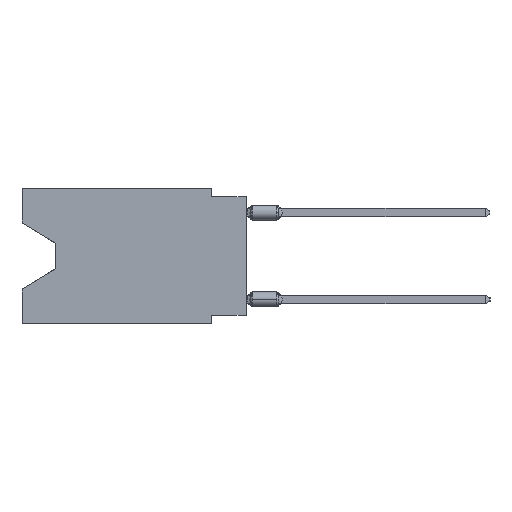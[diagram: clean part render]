
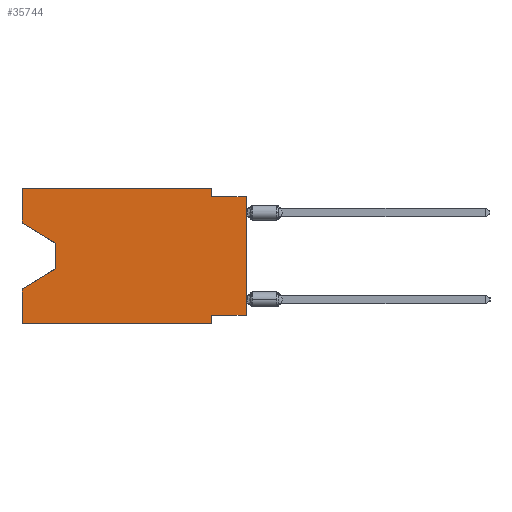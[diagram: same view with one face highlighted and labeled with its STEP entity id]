
A CAD part, left-side view. The second image highlights one B-rep face of the part: STEP entity #35744.
In plain terms, the highlighted planar face has unit normal (-1, 0, 0).
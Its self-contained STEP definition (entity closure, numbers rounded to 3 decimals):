
#128 = DIRECTION ( 'NONE',  ( 0., 1., 0. ) ) ;
#1043 = DIRECTION ( 'NONE',  ( 0., 0., 1. ) ) ;
#1381 = ORIENTED_EDGE ( 'NONE', *, *, #25218, .F. ) ;
#1422 = DIRECTION ( 'NONE',  ( 0., 0., 1. ) ) ;
#1975 = CARTESIAN_POINT ( 'NONE',  ( 0., 2.54, 0. ) ) ;
#2004 = CARTESIAN_POINT ( 'NONE',  ( 0., 16.383, -9.906 ) ) ;
#2198 = VERTEX_POINT ( 'NONE', #19059 ) ;
#2706 = VECTOR ( 'NONE', #7059, 1000. ) ;
#2719 = ORIENTED_EDGE ( 'NONE', *, *, #11180, .F. ) ;
#2769 = VECTOR ( 'NONE', #11578, 1000. ) ;
#6091 = EDGE_CURVE ( 'NONE', #43332, #20529, #32416, .T. ) ;
#7059 = DIRECTION ( 'NONE',  ( 0., -1., 0. ) ) ;
#7175 = VERTEX_POINT ( 'NONE', #13653 ) ;
#8090 = ORIENTED_EDGE ( 'NONE', *, *, #6091, .F. ) ;
#8791 = LINE ( 'NONE', #39538, #25114 ) ;
#9364 = PLANE ( 'NONE',  #44257 ) ;
#9762 = DIRECTION ( 'NONE',  ( 0., -0.855, -0.519 ) ) ;
#10087 = CARTESIAN_POINT ( 'NONE',  ( 0., 0., -0.635 ) ) ;
#10219 = ORIENTED_EDGE ( 'NONE', *, *, #27641, .F. ) ;
#10452 = EDGE_CURVE ( 'NONE', #34812, #7175, #15014, .T. ) ;
#10485 = ORIENTED_EDGE ( 'NONE', *, *, #10452, .F. ) ;
#10496 = VERTEX_POINT ( 'NONE', #26761 ) ;
#10949 = DIRECTION ( 'NONE',  ( 0., 0., -1. ) ) ;
#11180 = EDGE_CURVE ( 'NONE', #10496, #34812, #26831, .T. ) ;
#11578 = DIRECTION ( 'NONE',  ( 0., 0., 1. ) ) ;
#11816 = CARTESIAN_POINT ( 'NONE',  ( 0., 16.383, 0. ) ) ;
#11869 = CARTESIAN_POINT ( 'NONE',  ( 0., 13.97, -5.893 ) ) ;
#12240 = DIRECTION ( 'NONE',  ( 0., 0., -1. ) ) ;
#12267 = EDGE_CURVE ( 'NONE', #14804, #2198, #32508, .T. ) ;
#13176 = EDGE_CURVE ( 'NONE', #7175, #35821, #25823, .T. ) ;
#13653 = CARTESIAN_POINT ( 'NONE',  ( 0., 2.54, -0.635 ) ) ;
#14524 = EDGE_CURVE ( 'NONE', #14804, #10496, #8791, .T. ) ;
#14695 = LINE ( 'NONE', #29933, #27916 ) ;
#14804 = VERTEX_POINT ( 'NONE', #32775 ) ;
#14843 = ORIENTED_EDGE ( 'NONE', *, *, #35526, .T. ) ;
#15014 = LINE ( 'NONE', #19745, #48569 ) ;
#16143 = VECTOR ( 'NONE', #39251, 1000. ) ;
#16859 = CARTESIAN_POINT ( 'NONE',  ( 0., 2.54, -9.271 ) ) ;
#17497 = DIRECTION ( 'NONE',  ( 0., -1., 0. ) ) ;
#17853 = DIRECTION ( 'NONE',  ( 0., 0., -1. ) ) ;
#18412 = CARTESIAN_POINT ( 'NONE',  ( 0., 13.97, -5.893 ) ) ;
#18840 = CARTESIAN_POINT ( 'NONE',  ( 0., 16.383, 0. ) ) ;
#19059 = CARTESIAN_POINT ( 'NONE',  ( 0., 13.97, -4.013 ) ) ;
#19110 = VECTOR ( 'NONE', #128, 1000. ) ;
#19327 = DIRECTION ( 'NONE',  ( 0., -1., 0. ) ) ;
#19745 = CARTESIAN_POINT ( 'NONE',  ( 0., 2.54, 0. ) ) ;
#19930 = CARTESIAN_POINT ( 'NONE',  ( 0., 16.383, 0. ) ) ;
#20529 = VERTEX_POINT ( 'NONE', #24560 ) ;
#20582 = EDGE_LOOP ( 'NONE', ( #40039, #39672, #14843, #8090, #33492, #10219, #1381, #37770, #24499, #10485, #2719, #35408 ) ) ;
#20684 = CARTESIAN_POINT ( 'NONE',  ( 0., 2.54, -9.906 ) ) ;
#20751 = CARTESIAN_POINT ( 'NONE',  ( 0., 2.54, -9.906 ) ) ;
#21979 = VERTEX_POINT ( 'NONE', #23022 ) ;
#22090 = CARTESIAN_POINT ( 'NONE',  ( 0., 0., -0.635 ) ) ;
#22870 = CARTESIAN_POINT ( 'NONE',  ( 0., 0., -9.271 ) ) ;
#23022 = CARTESIAN_POINT ( 'NONE',  ( 0., 0., -9.271 ) ) ;
#24499 = ORIENTED_EDGE ( 'NONE', *, *, #13176, .F. ) ;
#24560 = CARTESIAN_POINT ( 'NONE',  ( 0., 16.383, -7.36 ) ) ;
#25114 = VECTOR ( 'NONE', #1043, 1000. ) ;
#25218 = EDGE_CURVE ( 'NONE', #21979, #26594, #49138, .T. ) ;
#25447 = VECTOR ( 'NONE', #19327, 1000. ) ;
#25823 = LINE ( 'NONE', #10087, #2706 ) ;
#26594 = VERTEX_POINT ( 'NONE', #16859 ) ;
#26761 = CARTESIAN_POINT ( 'NONE',  ( 0., 16.383, 0. ) ) ;
#26831 = LINE ( 'NONE', #11816, #25447 ) ;
#27616 = DIRECTION ( 'NONE',  ( 0., 0.855, -0.519 ) ) ;
#27641 = EDGE_CURVE ( 'NONE', #26594, #38222, #31993, .T. ) ;
#27778 = EDGE_CURVE ( 'NONE', #43332, #38222, #40493, .T. ) ;
#27916 = VECTOR ( 'NONE', #10949, 1000. ) ;
#29819 = CARTESIAN_POINT ( 'NONE',  ( 0., 16.383, -9.906 ) ) ;
#29933 = CARTESIAN_POINT ( 'NONE',  ( 0., 13.97, -4.013 ) ) ;
#30566 = LINE ( 'NONE', #45817, #2769 ) ;
#31354 = LINE ( 'NONE', #11869, #36268 ) ;
#31993 = LINE ( 'NONE', #20751, #16143 ) ;
#32101 = FACE_OUTER_BOUND ( 'NONE', #20582, .T. ) ;
#32416 = LINE ( 'NONE', #19930, #42876 ) ;
#32508 = LINE ( 'NONE', #48500, #44802 ) ;
#32519 = EDGE_CURVE ( 'NONE', #21979, #35821, #30566, .T. ) ;
#32775 = CARTESIAN_POINT ( 'NONE',  ( 0., 16.383, -2.546 ) ) ;
#33492 = ORIENTED_EDGE ( 'NONE', *, *, #27778, .T. ) ;
#34812 = VERTEX_POINT ( 'NONE', #1975 ) ;
#35408 = ORIENTED_EDGE ( 'NONE', *, *, #14524, .F. ) ;
#35526 = EDGE_CURVE ( 'NONE', #38280, #20529, #31354, .T. ) ;
#35744 = ADVANCED_FACE ( 'NONE', ( #32101 ), #9364, .F. ) ;
#35821 = VERTEX_POINT ( 'NONE', #22090 ) ;
#36268 = VECTOR ( 'NONE', #27616, 1000. ) ;
#36894 = VECTOR ( 'NONE', #17497, 1000. ) ;
#37770 = ORIENTED_EDGE ( 'NONE', *, *, #32519, .T. ) ;
#38222 = VERTEX_POINT ( 'NONE', #20684 ) ;
#38280 = VERTEX_POINT ( 'NONE', #18412 ) ;
#39251 = DIRECTION ( 'NONE',  ( 0., 0., -1. ) ) ;
#39538 = CARTESIAN_POINT ( 'NONE',  ( 0., 16.383, 0. ) ) ;
#39672 = ORIENTED_EDGE ( 'NONE', *, *, #48928, .T. ) ;
#40039 = ORIENTED_EDGE ( 'NONE', *, *, #12267, .T. ) ;
#40493 = LINE ( 'NONE', #2004, #36894 ) ;
#42876 = VECTOR ( 'NONE', #1422, 1000. ) ;
#43332 = VERTEX_POINT ( 'NONE', #29819 ) ;
#44257 = AXIS2_PLACEMENT_3D ( 'NONE', #18840, #48347, #17853 ) ;
#44802 = VECTOR ( 'NONE', #9762, 1000. ) ;
#45817 = CARTESIAN_POINT ( 'NONE',  ( 0., 0., 0. ) ) ;
#48347 = DIRECTION ( 'NONE',  ( 1., 0., 0. ) ) ;
#48500 = CARTESIAN_POINT ( 'NONE',  ( 0., 16.383, -2.546 ) ) ;
#48569 = VECTOR ( 'NONE', #12240, 1000. ) ;
#48928 = EDGE_CURVE ( 'NONE', #2198, #38280, #14695, .T. ) ;
#49138 = LINE ( 'NONE', #22870, #19110 ) ;
